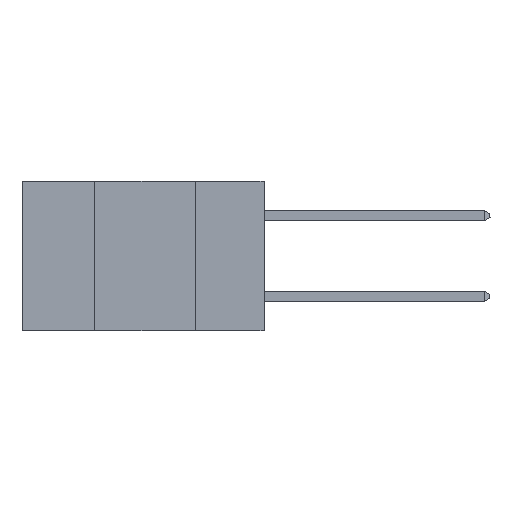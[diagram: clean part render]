
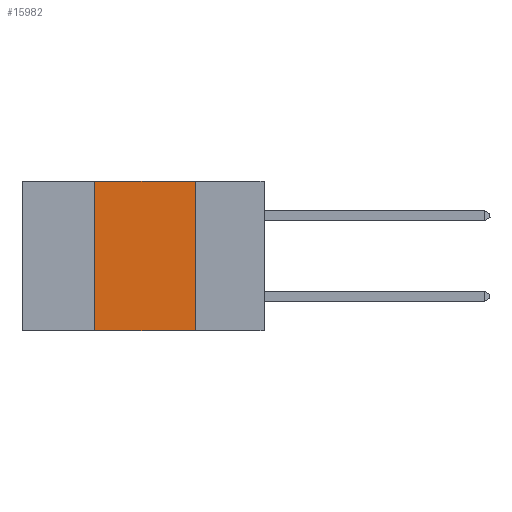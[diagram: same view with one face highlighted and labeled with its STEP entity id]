
A CAD part, left-side view. The second image highlights one B-rep face of the part: STEP entity #15982.
In plain terms, the highlighted planar face has unit normal (-1, 0, 0).
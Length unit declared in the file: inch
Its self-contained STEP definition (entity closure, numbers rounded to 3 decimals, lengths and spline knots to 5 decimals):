
#1689 = VERTEX_POINT ( 'NONE', #1779 ) ;
#1779 = CARTESIAN_POINT ( 'NONE',  ( 0., 0.17, 0. ) ) ;
#1799 = ORIENTED_EDGE ( 'NONE', *, *, #5707, .F. ) ;
#2131 = CARTESIAN_POINT ( 'NONE',  ( 0., 0.6, 0. ) ) ;
#3254 = VERTEX_POINT ( 'NONE', #20965 ) ;
#4277 = CARTESIAN_POINT ( 'NONE',  ( 0., 0.42, 0. ) ) ;
#5364 = DIRECTION ( 'NONE',  ( 0., 0., 1. ) ) ;
#5629 = DIRECTION ( 'NONE',  ( 1., 0., 0. ) ) ;
#5707 = EDGE_CURVE ( 'NONE', #1689, #3254, #28891, .T. ) ;
#6084 = ORIENTED_EDGE ( 'NONE', *, *, #17314, .T. ) ;
#7214 = ORIENTED_EDGE ( 'NONE', *, *, #19959, .F. ) ;
#9477 = AXIS2_PLACEMENT_3D ( 'NONE', #25076, #5629, #27414 ) ;
#11124 = VECTOR ( 'NONE', #23543, 39.37008 ) ;
#11903 = LINE ( 'NONE', #2131, #11124 ) ;
#12351 = ORIENTED_EDGE ( 'NONE', *, *, #20792, .F. ) ;
#13230 = CARTESIAN_POINT ( 'NONE',  ( 0., 0.6, -0.37 ) ) ;
#15982 = ADVANCED_FACE ( 'NONE', ( #18202 ), #22549, .F. ) ;
#17314 = EDGE_CURVE ( 'NONE', #19196, #3254, #26470, .T. ) ;
#17544 = VECTOR ( 'NONE', #5364, 39.37008 ) ;
#18202 = FACE_OUTER_BOUND ( 'NONE', #28449, .T. ) ;
#19196 = VERTEX_POINT ( 'NONE', #21261 ) ;
#19654 = VECTOR ( 'NONE', #27607, 39.37008 ) ;
#19823 = CARTESIAN_POINT ( 'NONE',  ( 0., 0.17, 0. ) ) ;
#19959 = EDGE_CURVE ( 'NONE', #23373, #1689, #11903, .T. ) ;
#20610 = VECTOR ( 'NONE', #24682, 39.37008 ) ;
#20792 = EDGE_CURVE ( 'NONE', #19196, #23373, #24716, .T. ) ;
#20965 = CARTESIAN_POINT ( 'NONE',  ( 0., 0.17, -0.37 ) ) ;
#21261 = CARTESIAN_POINT ( 'NONE',  ( 0., 0.42, -0.37 ) ) ;
#22549 = PLANE ( 'NONE',  #9477 ) ;
#23373 = VERTEX_POINT ( 'NONE', #4277 ) ;
#23543 = DIRECTION ( 'NONE',  ( 0., -1., 0. ) ) ;
#24682 = DIRECTION ( 'NONE',  ( 0., 0., -1. ) ) ;
#24716 = LINE ( 'NONE', #29879, #17544 ) ;
#25076 = CARTESIAN_POINT ( 'NONE',  ( 0., 0.6, 0. ) ) ;
#26470 = LINE ( 'NONE', #13230, #19654 ) ;
#27414 = DIRECTION ( 'NONE',  ( 0., 0., -1. ) ) ;
#27607 = DIRECTION ( 'NONE',  ( 0., -1., 0. ) ) ;
#28449 = EDGE_LOOP ( 'NONE', ( #1799, #7214, #12351, #6084 ) ) ;
#28891 = LINE ( 'NONE', #19823, #20610 ) ;
#29879 = CARTESIAN_POINT ( 'NONE',  ( 0., 0.42, 0. ) ) ;
